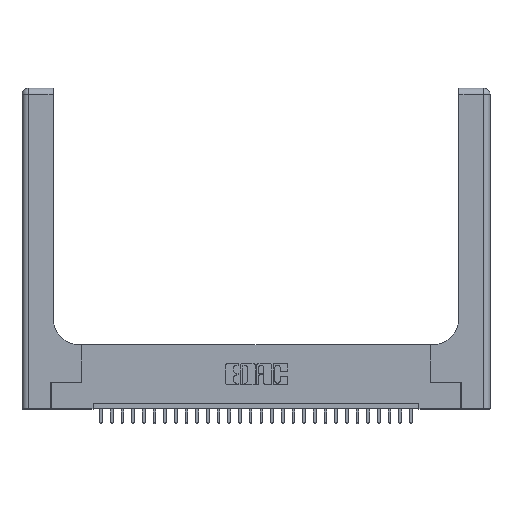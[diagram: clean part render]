
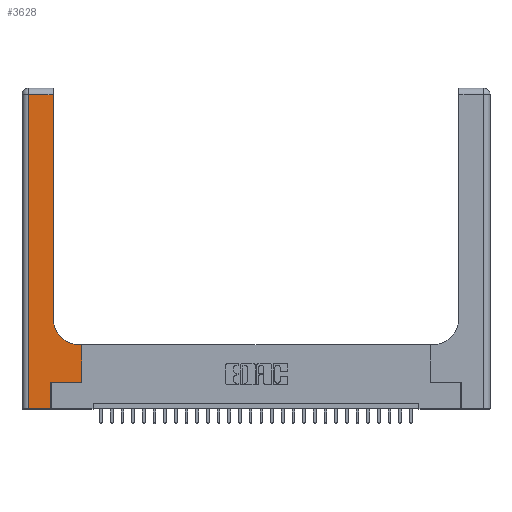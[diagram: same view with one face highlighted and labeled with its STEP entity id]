
A CAD part, top view. The second image highlights one B-rep face of the part: STEP entity #3628.
In plain terms, the highlighted planar face has unit normal (0, 0, 1).
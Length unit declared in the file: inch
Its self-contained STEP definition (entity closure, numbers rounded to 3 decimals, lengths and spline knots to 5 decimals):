
#178 = EDGE_CURVE ( 'NONE', #19186, #9114, #27919, .T. ) ;
#282 = CARTESIAN_POINT ( 'NONE',  ( 0.269, 0., 0.37 ) ) ;
#677 = DIRECTION ( 'NONE',  ( 0., 1., 0. ) ) ;
#1111 = CARTESIAN_POINT ( 'NONE',  ( 0.2915, 0.85, 0.37 ) ) ;
#1758 = CARTESIAN_POINT ( 'NONE',  ( 0., 3., 0.37 ) ) ;
#3233 = VERTEX_POINT ( 'NONE', #25705 ) ;
#3628 = ADVANCED_FACE ( 'NONE', ( #15993 ), #29403, .F. ) ;
#4207 = DIRECTION ( 'NONE',  ( -1., 0., 0. ) ) ;
#5062 = ORIENTED_EDGE ( 'NONE', *, *, #23986, .T. ) ;
#5064 = VECTOR ( 'NONE', #5434, 39.37008 ) ;
#5434 = DIRECTION ( 'NONE',  ( 0., -1., 0. ) ) ;
#5693 = CARTESIAN_POINT ( 'NONE',  ( 0.06, 0., 0.37 ) ) ;
#5914 = VECTOR ( 'NONE', #20069, 39.37008 ) ;
#5920 = CARTESIAN_POINT ( 'NONE',  ( 0.5415, 0.85, 0.37 ) ) ;
#5963 = LINE ( 'NONE', #7047, #15862 ) ;
#6302 = DIRECTION ( 'NONE',  ( 0., 0., -1. ) ) ;
#6523 = DIRECTION ( 'NONE',  ( 0., 0., -1. ) ) ;
#6576 = CARTESIAN_POINT ( 'NONE',  ( 0.2915, 0.6, 0.37 ) ) ;
#6896 = CARTESIAN_POINT ( 'NONE',  ( 0.269, 0.25, 0.37 ) ) ;
#7047 = CARTESIAN_POINT ( 'NONE',  ( 0.2915, 3., 0.37 ) ) ;
#7517 = VECTOR ( 'NONE', #9245, 39.37008 ) ;
#7788 = AXIS2_PLACEMENT_3D ( 'NONE', #5920, #6523, #24301 ) ;
#8818 = VERTEX_POINT ( 'NONE', #5693 ) ;
#9114 = VERTEX_POINT ( 'NONE', #24163 ) ;
#9245 = DIRECTION ( 'NONE',  ( -1., 0., 0. ) ) ;
#9573 = CARTESIAN_POINT ( 'NONE',  ( 0.06, 2.94, 0.37 ) ) ;
#9919 = ORIENTED_EDGE ( 'NONE', *, *, #12065, .T. ) ;
#10147 = VECTOR ( 'NONE', #24862, 39.37008 ) ;
#10224 = ORIENTED_EDGE ( 'NONE', *, *, #29235, .T. ) ;
#10817 = EDGE_LOOP ( 'NONE', ( #11469, #5062, #26693, #9919, #10224, #19368, #26840, #14282, #18501 ) ) ;
#11469 = ORIENTED_EDGE ( 'NONE', *, *, #12439, .T. ) ;
#11909 = CARTESIAN_POINT ( 'NONE',  ( 0., 0., 0.37 ) ) ;
#12065 = EDGE_CURVE ( 'NONE', #8818, #15110, #22258, .T. ) ;
#12439 = EDGE_CURVE ( 'NONE', #26636, #27699, #5963, .T. ) ;
#12594 = LINE ( 'NONE', #15565, #10147 ) ;
#13486 = VECTOR ( 'NONE', #4207, 39.37008 ) ;
#13600 = CIRCLE ( 'NONE', #7788, 0.25 ) ;
#14199 = LINE ( 'NONE', #6576, #13486 ) ;
#14282 = ORIENTED_EDGE ( 'NONE', *, *, #26125, .T. ) ;
#14606 = EDGE_CURVE ( 'NONE', #9114, #18106, #12594, .T. ) ;
#15110 = VERTEX_POINT ( 'NONE', #26430 ) ;
#15565 = CARTESIAN_POINT ( 'NONE',  ( 0.5585, 0.25, 0.37 ) ) ;
#15621 = EDGE_CURVE ( 'NONE', #3233, #26636, #13600, .T. ) ;
#15862 = VECTOR ( 'NONE', #20416, 39.37008 ) ;
#15993 = FACE_OUTER_BOUND ( 'NONE', #10817, .T. ) ;
#16170 = VECTOR ( 'NONE', #18630, 39.37008 ) ;
#17956 = LINE ( 'NONE', #282, #22266 ) ;
#18106 = VERTEX_POINT ( 'NONE', #28292 ) ;
#18501 = ORIENTED_EDGE ( 'NONE', *, *, #15621, .T. ) ;
#18630 = DIRECTION ( 'NONE',  ( 1., 0., 0. ) ) ;
#19186 = VERTEX_POINT ( 'NONE', #23726 ) ;
#19368 = ORIENTED_EDGE ( 'NONE', *, *, #178, .T. ) ;
#20069 = DIRECTION ( 'NONE',  ( 1., 0., 0. ) ) ;
#20416 = DIRECTION ( 'NONE',  ( 0., 1., 0. ) ) ;
#22159 = DIRECTION ( 'NONE',  ( -1., 0., 0. ) ) ;
#22258 = LINE ( 'NONE', #11909, #16170 ) ;
#22266 = VECTOR ( 'NONE', #677, 39.37008 ) ;
#22642 = CARTESIAN_POINT ( 'NONE',  ( 0., 2.94, 0.37 ) ) ;
#23183 = LINE ( 'NONE', #24548, #5064 ) ;
#23726 = CARTESIAN_POINT ( 'NONE',  ( 0.269, 0.25, 0.37 ) ) ;
#23933 = EDGE_CURVE ( 'NONE', #28521, #8818, #23183, .T. ) ;
#23986 = EDGE_CURVE ( 'NONE', #27699, #28521, #28132, .T. ) ;
#24163 = CARTESIAN_POINT ( 'NONE',  ( 0.5585, 0.25, 0.37 ) ) ;
#24301 = DIRECTION ( 'NONE',  ( 1., 0., 0. ) ) ;
#24548 = CARTESIAN_POINT ( 'NONE',  ( 0.06, 3., 0.37 ) ) ;
#24577 = AXIS2_PLACEMENT_3D ( 'NONE', #1758, #6302, #22159 ) ;
#24862 = DIRECTION ( 'NONE',  ( 0., 1., 0. ) ) ;
#25705 = CARTESIAN_POINT ( 'NONE',  ( 0.5415, 0.6, 0.37 ) ) ;
#26125 = EDGE_CURVE ( 'NONE', #18106, #3233, #14199, .T. ) ;
#26374 = CARTESIAN_POINT ( 'NONE',  ( 0.2915, 2.94, 0.37 ) ) ;
#26430 = CARTESIAN_POINT ( 'NONE',  ( 0.269, 0., 0.37 ) ) ;
#26636 = VERTEX_POINT ( 'NONE', #1111 ) ;
#26693 = ORIENTED_EDGE ( 'NONE', *, *, #23933, .T. ) ;
#26840 = ORIENTED_EDGE ( 'NONE', *, *, #14606, .T. ) ;
#27699 = VERTEX_POINT ( 'NONE', #26374 ) ;
#27919 = LINE ( 'NONE', #6896, #5914 ) ;
#28132 = LINE ( 'NONE', #22642, #7517 ) ;
#28292 = CARTESIAN_POINT ( 'NONE',  ( 0.5585, 0.6, 0.37 ) ) ;
#28521 = VERTEX_POINT ( 'NONE', #9573 ) ;
#29235 = EDGE_CURVE ( 'NONE', #15110, #19186, #17956, .T. ) ;
#29403 = PLANE ( 'NONE',  #24577 ) ;
